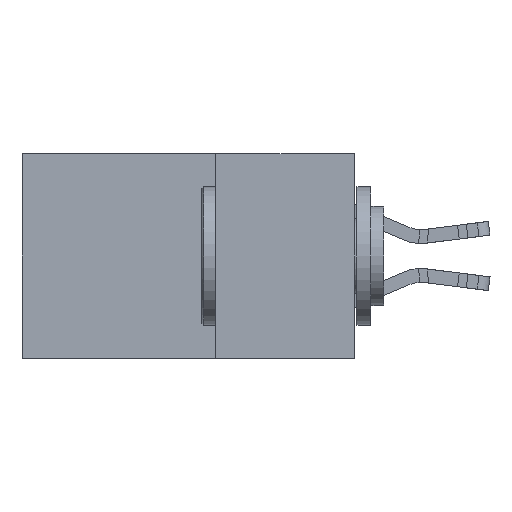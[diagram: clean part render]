
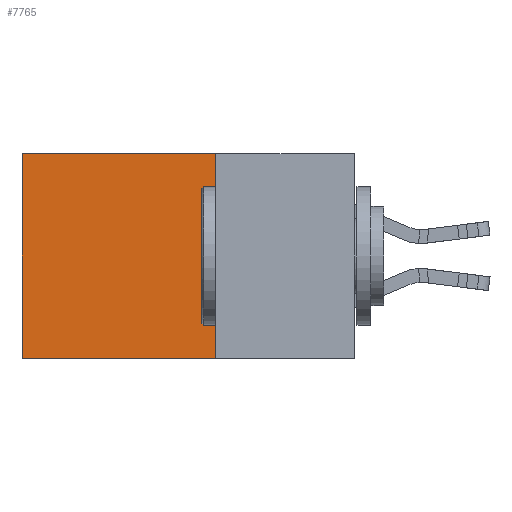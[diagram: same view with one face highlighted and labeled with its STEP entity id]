
A CAD part, left-side view. The second image highlights one B-rep face of the part: STEP entity #7765.
In plain terms, the highlighted planar face has unit normal (-1, 0, 0).
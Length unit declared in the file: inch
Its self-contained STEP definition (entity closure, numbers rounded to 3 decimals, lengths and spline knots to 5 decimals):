
#514 = ORIENTED_EDGE ( 'NONE', *, *, #1739, .F. ) ;
#580 = CARTESIAN_POINT ( 'NONE',  ( 0.298, 0.25, 0. ) ) ;
#1233 = FACE_OUTER_BOUND ( 'NONE', #30649, .T. ) ;
#1739 = EDGE_CURVE ( 'NONE', #25515, #11667, #23263, .T. ) ;
#2765 = EDGE_CURVE ( 'NONE', #11667, #27163, #30096, .T. ) ;
#4177 = AXIS2_PLACEMENT_3D ( 'NONE', #4280, #31320, #9514 ) ;
#4280 = CARTESIAN_POINT ( 'NONE',  ( 0.298, 0.25, 0. ) ) ;
#4532 = LINE ( 'NONE', #31458, #29036 ) ;
#4821 = DIRECTION ( 'NONE',  ( 0., 0., -1. ) ) ;
#6578 = LINE ( 'NONE', #12003, #22667 ) ;
#7765 = ADVANCED_FACE ( 'NONE', ( #1233 ), #11799, .F. ) ;
#8291 = VERTEX_POINT ( 'NONE', #24766 ) ;
#8776 = VECTOR ( 'NONE', #4821, 39.37008 ) ;
#9514 = DIRECTION ( 'NONE',  ( 0., 0., -1. ) ) ;
#11235 = DIRECTION ( 'NONE',  ( 0., 1., 0. ) ) ;
#11667 = VERTEX_POINT ( 'NONE', #23075 ) ;
#11799 = PLANE ( 'NONE',  #4177 ) ;
#12003 = CARTESIAN_POINT ( 'NONE',  ( 0.298, 0.6, 0. ) ) ;
#13001 = EDGE_CURVE ( 'NONE', #8291, #27163, #6578, .T. ) ;
#13914 = ORIENTED_EDGE ( 'NONE', *, *, #2765, .F. ) ;
#15231 = VECTOR ( 'NONE', #11235, 39.37008 ) ;
#17306 = ORIENTED_EDGE ( 'NONE', *, *, #13001, .T. ) ;
#21541 = DIRECTION ( 'NONE',  ( 0., 1., 0. ) ) ;
#22667 = VECTOR ( 'NONE', #24164, 39.37008 ) ;
#23075 = CARTESIAN_POINT ( 'NONE',  ( 0.298, 0.25, -0.37 ) ) ;
#23263 = LINE ( 'NONE', #26574, #8776 ) ;
#23498 = CARTESIAN_POINT ( 'NONE',  ( 0.298, 0.25, -0.37 ) ) ;
#24164 = DIRECTION ( 'NONE',  ( 0., 0., -1. ) ) ;
#24766 = CARTESIAN_POINT ( 'NONE',  ( 0.298, 0.6, 0. ) ) ;
#25515 = VERTEX_POINT ( 'NONE', #580 ) ;
#25549 = ORIENTED_EDGE ( 'NONE', *, *, #28844, .T. ) ;
#26574 = CARTESIAN_POINT ( 'NONE',  ( 0.298, 0.25, 0. ) ) ;
#27163 = VERTEX_POINT ( 'NONE', #27672 ) ;
#27672 = CARTESIAN_POINT ( 'NONE',  ( 0.298, 0.6, -0.37 ) ) ;
#28844 = EDGE_CURVE ( 'NONE', #25515, #8291, #4532, .T. ) ;
#29036 = VECTOR ( 'NONE', #21541, 39.37008 ) ;
#30096 = LINE ( 'NONE', #23498, #15231 ) ;
#30649 = EDGE_LOOP ( 'NONE', ( #17306, #13914, #514, #25549 ) ) ;
#31320 = DIRECTION ( 'NONE',  ( 1., 0., 0. ) ) ;
#31458 = CARTESIAN_POINT ( 'NONE',  ( 0.298, 0.25, 0. ) ) ;
